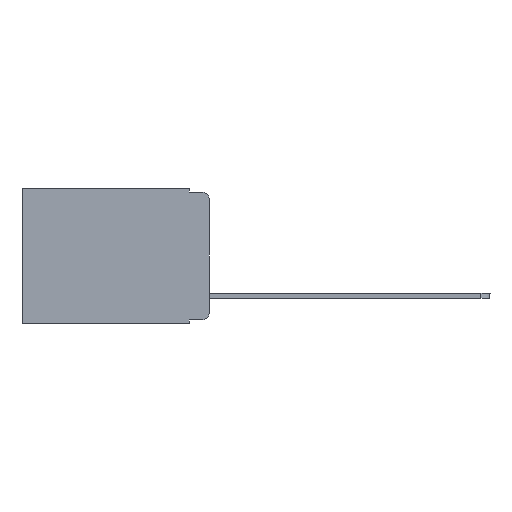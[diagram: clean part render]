
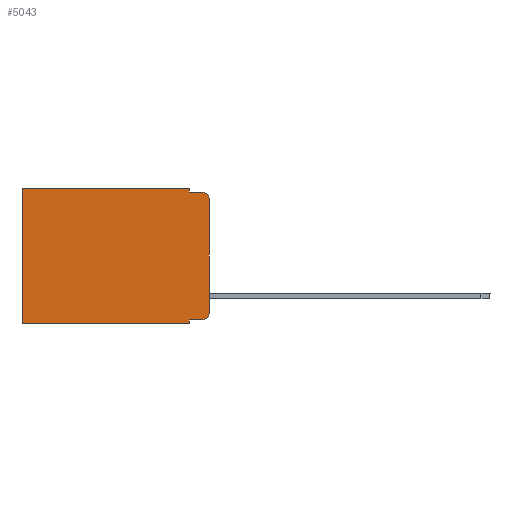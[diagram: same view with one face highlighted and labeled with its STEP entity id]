
A CAD part, left-side view. The second image highlights one B-rep face of the part: STEP entity #5043.
In plain terms, the highlighted planar face has unit normal (-1, 0, 0).
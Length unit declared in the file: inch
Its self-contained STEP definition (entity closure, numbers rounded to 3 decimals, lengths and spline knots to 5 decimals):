
#145 = DIRECTION ( 'NONE',  ( 0., -1., 0. ) ) ;
#228 = EDGE_CURVE ( 'NONE', #8420, #907, #9852, .T. ) ;
#246 = AXIS2_PLACEMENT_3D ( 'NONE', #5781, #1009, #11364 ) ;
#351 = ORIENTED_EDGE ( 'NONE', *, *, #7375, .F. ) ;
#432 = CARTESIAN_POINT ( 'NONE',  ( 0.298, 0.051, 0. ) ) ;
#480 = EDGE_CURVE ( 'NONE', #6230, #7381, #12073, .T. ) ;
#493 = DIRECTION ( 'NONE',  ( 0., -1., 0. ) ) ;
#501 = VECTOR ( 'NONE', #145, 39.37008 ) ;
#692 = VECTOR ( 'NONE', #493, 39.37008 ) ;
#788 = CARTESIAN_POINT ( 'NONE',  ( 0.298, 0.473, -0.343 ) ) ;
#907 = VERTEX_POINT ( 'NONE', #788 ) ;
#915 = VECTOR ( 'NONE', #3949, 39.37008 ) ;
#1009 = DIRECTION ( 'NONE',  ( -1., 0., 0. ) ) ;
#1047 = VECTOR ( 'NONE', #4729, 39.37008 ) ;
#1147 = CARTESIAN_POINT ( 'NONE',  ( 0.298, 0.473, 0. ) ) ;
#1198 = ORIENTED_EDGE ( 'NONE', *, *, #228, .F. ) ;
#1373 = EDGE_LOOP ( 'NONE', ( #8399, #10316, #8164, #9540, #9577, #2371, #1198, #351, #5152, #8141 ) ) ;
#1381 = VERTEX_POINT ( 'NONE', #9875 ) ;
#1399 = DIRECTION ( 'NONE',  ( -1., 0., 0. ) ) ;
#1588 = DIRECTION ( 'NONE',  ( 0., 1., 0. ) ) ;
#1831 = CIRCLE ( 'NONE', #246, 0.02 ) ;
#1892 = AXIS2_PLACEMENT_3D ( 'NONE', #1962, #1399, #9886 ) ;
#1962 = CARTESIAN_POINT ( 'NONE',  ( 0.298, 0.02, -0.03 ) ) ;
#2034 = CARTESIAN_POINT ( 'NONE',  ( 0.298, 0., -0.03 ) ) ;
#2183 = VERTEX_POINT ( 'NONE', #2034 ) ;
#2371 = ORIENTED_EDGE ( 'NONE', *, *, #4701, .T. ) ;
#2685 = EDGE_CURVE ( 'NONE', #2183, #10293, #10402, .T. ) ;
#2822 = CARTESIAN_POINT ( 'NONE',  ( 0.298, 0., 0. ) ) ;
#2922 = CARTESIAN_POINT ( 'NONE',  ( 0.298, 0., -0.313 ) ) ;
#3239 = DIRECTION ( 'NONE',  ( 0., 0., -1. ) ) ;
#3354 = CARTESIAN_POINT ( 'NONE',  ( 0.298, 0.051, 0. ) ) ;
#3437 = DIRECTION ( 'NONE',  ( 0., 0., -1. ) ) ;
#3483 = CARTESIAN_POINT ( 'NONE',  ( 0.298, 0., 0. ) ) ;
#3628 = LINE ( 'NONE', #9711, #692 ) ;
#3763 = DIRECTION ( 'NONE',  ( 1., 0., 0. ) ) ;
#3866 = EDGE_CURVE ( 'NONE', #4583, #1381, #4162, .T. ) ;
#3890 = EDGE_CURVE ( 'NONE', #1381, #4343, #1831, .T. ) ;
#3949 = DIRECTION ( 'NONE',  ( 0., 0., -1. ) ) ;
#4162 = LINE ( 'NONE', #7664, #501 ) ;
#4343 = VERTEX_POINT ( 'NONE', #2922 ) ;
#4456 = VERTEX_POINT ( 'NONE', #1147 ) ;
#4583 = VERTEX_POINT ( 'NONE', #4734 ) ;
#4701 = EDGE_CURVE ( 'NONE', #4456, #907, #6214, .T. ) ;
#4729 = DIRECTION ( 'NONE',  ( 0., 0., -1. ) ) ;
#4734 = CARTESIAN_POINT ( 'NONE',  ( 0.298, 0.051, -0.333 ) ) ;
#5043 = ADVANCED_FACE ( 'NONE', ( #9428 ), #5543, .F. ) ;
#5152 = ORIENTED_EDGE ( 'NONE', *, *, #3866, .T. ) ;
#5543 = PLANE ( 'NONE',  #10953 ) ;
#5781 = CARTESIAN_POINT ( 'NONE',  ( 0.298, 0.02, -0.313 ) ) ;
#6214 = LINE ( 'NONE', #9626, #915 ) ;
#6230 = VERTEX_POINT ( 'NONE', #10723 ) ;
#6386 = LINE ( 'NONE', #3483, #9189 ) ;
#6431 = DIRECTION ( 'NONE',  ( 0., 0., -1. ) ) ;
#6738 = EDGE_CURVE ( 'NONE', #7381, #10293, #3628, .T. ) ;
#7192 = CARTESIAN_POINT ( 'NONE',  ( 0.298, 0., 0. ) ) ;
#7203 = VECTOR ( 'NONE', #10288, 39.37008 ) ;
#7353 = CARTESIAN_POINT ( 'NONE',  ( 0.298, 0., -0.343 ) ) ;
#7375 = EDGE_CURVE ( 'NONE', #4583, #8420, #7717, .T. ) ;
#7381 = VERTEX_POINT ( 'NONE', #9956 ) ;
#7504 = EDGE_CURVE ( 'NONE', #6230, #4456, #6386, .T. ) ;
#7664 = CARTESIAN_POINT ( 'NONE',  ( 0.298, 0.051, -0.333 ) ) ;
#7717 = LINE ( 'NONE', #432, #9640 ) ;
#8141 = ORIENTED_EDGE ( 'NONE', *, *, #3890, .T. ) ;
#8164 = ORIENTED_EDGE ( 'NONE', *, *, #6738, .F. ) ;
#8197 = CARTESIAN_POINT ( 'NONE',  ( 0.298, 0.051, -0.343 ) ) ;
#8399 = ORIENTED_EDGE ( 'NONE', *, *, #9978, .F. ) ;
#8420 = VERTEX_POINT ( 'NONE', #8197 ) ;
#8823 = CARTESIAN_POINT ( 'NONE',  ( 0.298, 0.02, -0.01 ) ) ;
#8957 = VECTOR ( 'NONE', #3437, 39.37008 ) ;
#9189 = VECTOR ( 'NONE', #1588, 39.37008 ) ;
#9428 = FACE_OUTER_BOUND ( 'NONE', #1373, .T. ) ;
#9540 = ORIENTED_EDGE ( 'NONE', *, *, #480, .F. ) ;
#9577 = ORIENTED_EDGE ( 'NONE', *, *, #7504, .T. ) ;
#9586 = LINE ( 'NONE', #7192, #1047 ) ;
#9626 = CARTESIAN_POINT ( 'NONE',  ( 0.298, 0.473, 0. ) ) ;
#9640 = VECTOR ( 'NONE', #3239, 39.37008 ) ;
#9711 = CARTESIAN_POINT ( 'NONE',  ( 0.298, 0.051, -0.01 ) ) ;
#9852 = LINE ( 'NONE', #7353, #7203 ) ;
#9875 = CARTESIAN_POINT ( 'NONE',  ( 0.298, 0.02, -0.333 ) ) ;
#9886 = DIRECTION ( 'NONE',  ( 0., 0., -1. ) ) ;
#9956 = CARTESIAN_POINT ( 'NONE',  ( 0.298, 0.051, -0.01 ) ) ;
#9978 = EDGE_CURVE ( 'NONE', #2183, #4343, #9586, .T. ) ;
#10288 = DIRECTION ( 'NONE',  ( 0., 1., 0. ) ) ;
#10293 = VERTEX_POINT ( 'NONE', #8823 ) ;
#10316 = ORIENTED_EDGE ( 'NONE', *, *, #2685, .T. ) ;
#10402 = CIRCLE ( 'NONE', #1892, 0.02 ) ;
#10723 = CARTESIAN_POINT ( 'NONE',  ( 0.298, 0.051, 0. ) ) ;
#10953 = AXIS2_PLACEMENT_3D ( 'NONE', #2822, #3763, #6431 ) ;
#11364 = DIRECTION ( 'NONE',  ( 0., 0., -1. ) ) ;
#12073 = LINE ( 'NONE', #3354, #8957 ) ;
